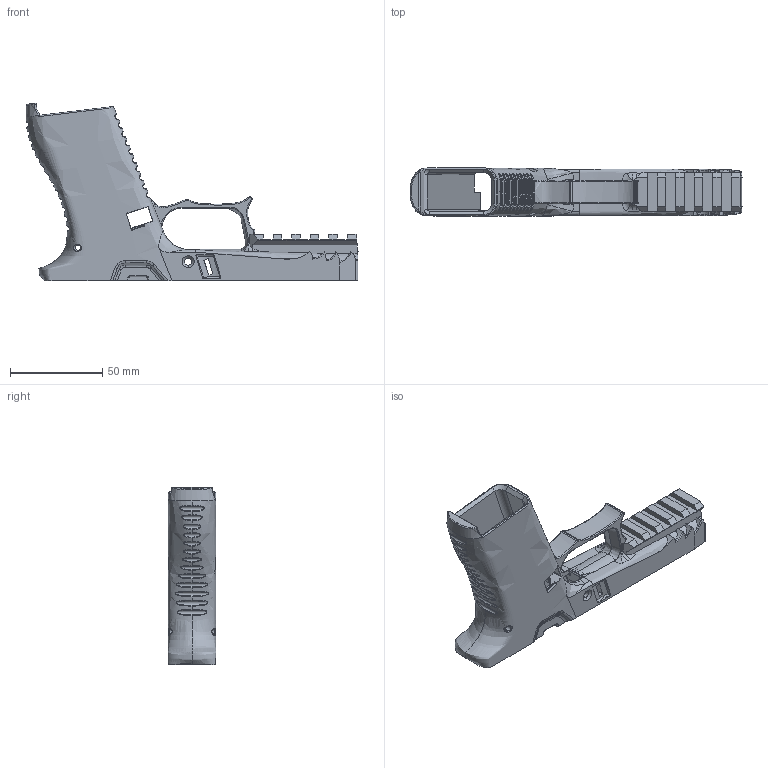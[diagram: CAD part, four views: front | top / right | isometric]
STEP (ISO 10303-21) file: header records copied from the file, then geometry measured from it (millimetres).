
FILE_DESCRIPTION (( 'STEP AP203' ), '1' );
FILE_NAME ('E48 Super Smooth FDM.STEP', '2020-12-17T02:04:41', ( '' ), ( '' ), 'SwSTEP 2.0', 'SolidWorks 2016', '' );
FILE_SCHEMA (( 'CONFIG_CONTROL_DESIGN' ));
Products named in the file (1): E48 Super Smooth FDM
Bounding box: 179.61 x 25.9 x 95.92 mm (x, y, z)
Volume: 75071.4 mm3; surface area: 41998.7 mm2
Topology: 1 solids, 1 shells, 1084 faces, 2942 edges, 1817 vertices
Faces by surface type: bspline 443, cylinder 363, plane 236, torus 26, cone 12, sphere 4
Entity records: 73637 total; most frequent: CARTESIAN_POINT 50990, ORIENTED_EDGE 5810, DIRECTION 3160, EDGE_CURVE 2905, VERTEX_POINT 1817, B_SPLINE_CURVE_WITH_KNOTS 1418, AXIS2_PLACEMENT_3D 1140, EDGE_LOOP 1100
